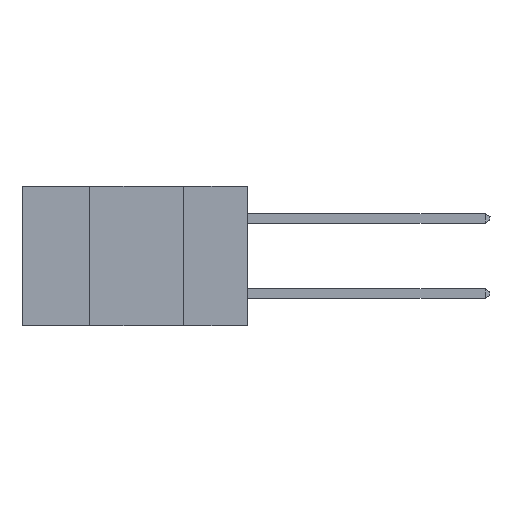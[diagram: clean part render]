
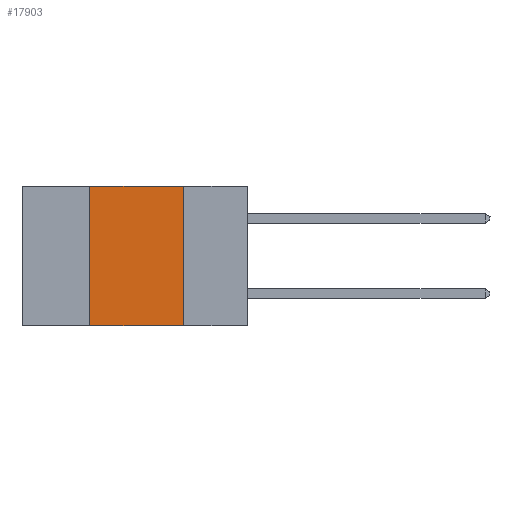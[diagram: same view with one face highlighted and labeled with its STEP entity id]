
A CAD part, left-side view. The second image highlights one B-rep face of the part: STEP entity #17903.
In plain terms, the highlighted planar face has unit normal (-1, 0, 0).
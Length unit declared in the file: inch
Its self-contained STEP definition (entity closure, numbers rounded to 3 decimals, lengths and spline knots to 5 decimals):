
#3202 = LINE ( 'NONE', #11836, #21058 ) ;
#3219 = VERTEX_POINT ( 'NONE', #17814 ) ;
#3295 = VERTEX_POINT ( 'NONE', #16642 ) ;
#6573 = DIRECTION ( 'NONE',  ( 0., 0., -1. ) ) ;
#7468 = VERTEX_POINT ( 'NONE', #18194 ) ;
#7930 = EDGE_CURVE ( 'NONE', #3295, #7468, #17474, .T. ) ;
#8249 = DIRECTION ( 'NONE',  ( 0., -1., 0. ) ) ;
#8708 = VECTOR ( 'NONE', #6573, 39.37008 ) ;
#11332 = EDGE_LOOP ( 'NONE', ( #22285, #12592, #19295, #13006 ) ) ;
#11836 = CARTESIAN_POINT ( 'NONE',  ( 0., 0.6, -0.37 ) ) ;
#12592 = ORIENTED_EDGE ( 'NONE', *, *, #12942, .F. ) ;
#12861 = VECTOR ( 'NONE', #17079, 39.37008 ) ;
#12942 = EDGE_CURVE ( 'NONE', #7468, #3219, #21508, .T. ) ;
#13006 = ORIENTED_EDGE ( 'NONE', *, *, #17205, .T. ) ;
#13321 = DIRECTION ( 'NONE',  ( 1., 0., 0. ) ) ;
#13861 = CARTESIAN_POINT ( 'NONE',  ( 0., 0.17, -0.37 ) ) ;
#14035 = AXIS2_PLACEMENT_3D ( 'NONE', #16727, #13321, #20263 ) ;
#14197 = LINE ( 'NONE', #17024, #8708 ) ;
#14769 = VECTOR ( 'NONE', #8249, 39.37008 ) ;
#14989 = PLANE ( 'NONE',  #14035 ) ;
#15352 = CARTESIAN_POINT ( 'NONE',  ( 0., 0.42, 0. ) ) ;
#16642 = CARTESIAN_POINT ( 'NONE',  ( 0., 0.42, -0.37 ) ) ;
#16727 = CARTESIAN_POINT ( 'NONE',  ( 0., 0.6, 0. ) ) ;
#17024 = CARTESIAN_POINT ( 'NONE',  ( 0., 0.17, 0. ) ) ;
#17073 = VERTEX_POINT ( 'NONE', #13861 ) ;
#17079 = DIRECTION ( 'NONE',  ( 0., 0., 1. ) ) ;
#17205 = EDGE_CURVE ( 'NONE', #3295, #17073, #3202, .T. ) ;
#17474 = LINE ( 'NONE', #15352, #12861 ) ;
#17814 = CARTESIAN_POINT ( 'NONE',  ( 0., 0.17, 0. ) ) ;
#17903 = ADVANCED_FACE ( 'NONE', ( #21803 ), #14989, .F. ) ;
#18035 = EDGE_CURVE ( 'NONE', #3219, #17073, #14197, .T. ) ;
#18194 = CARTESIAN_POINT ( 'NONE',  ( 0., 0.42, 0. ) ) ;
#19295 = ORIENTED_EDGE ( 'NONE', *, *, #7930, .F. ) ;
#20263 = DIRECTION ( 'NONE',  ( 0., 0., -1. ) ) ;
#20421 = CARTESIAN_POINT ( 'NONE',  ( 0., 0.6, 0. ) ) ;
#20983 = DIRECTION ( 'NONE',  ( 0., -1., 0. ) ) ;
#21058 = VECTOR ( 'NONE', #20983, 39.37008 ) ;
#21508 = LINE ( 'NONE', #20421, #14769 ) ;
#21803 = FACE_OUTER_BOUND ( 'NONE', #11332, .T. ) ;
#22285 = ORIENTED_EDGE ( 'NONE', *, *, #18035, .F. ) ;
